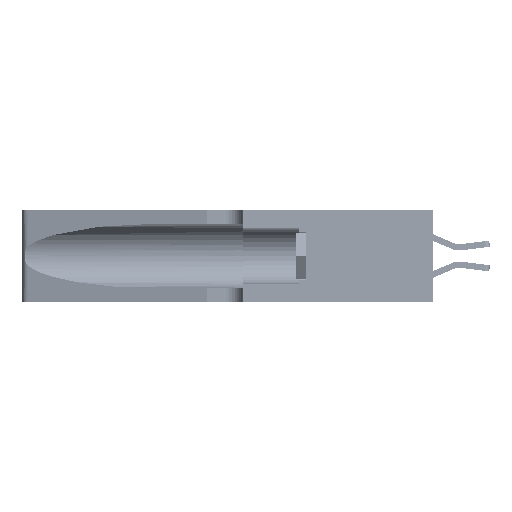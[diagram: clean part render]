
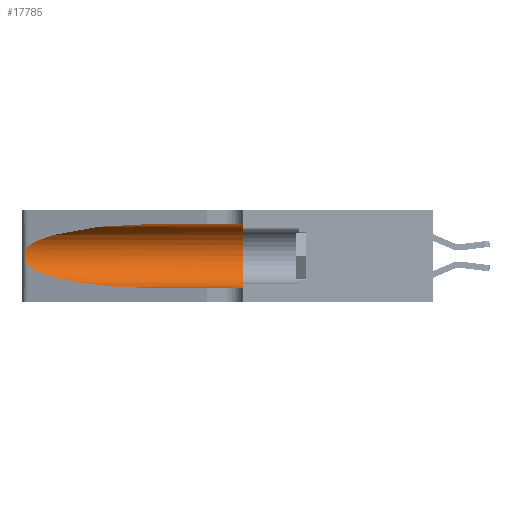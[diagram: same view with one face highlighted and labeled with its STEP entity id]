
A CAD part, left-side view. The second image highlights one B-rep face of the part: STEP entity #17785.
In plain terms, the highlighted cylindrical face has radius 3.308 mm (diameter 6.617 mm), a partial arc.
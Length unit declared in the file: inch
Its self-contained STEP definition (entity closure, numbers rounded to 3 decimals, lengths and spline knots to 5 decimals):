
#427 = CARTESIAN_POINT ( 'NONE',  ( 0.1305, 0.72297, 0.31525 ) ) ;
#527 = CARTESIAN_POINT ( 'NONE',  ( 0.25555, 1.22994, 0.2215 ) ) ;
#668 = CARTESIAN_POINT ( 'NONE',  ( 0.25639, 1.23186, 0.15144 ) ) ;
#2680 = ORIENTED_EDGE ( 'NONE', *, *, #5935, .T. ) ;
#2803 = LINE ( 'NONE', #15591, #28106 ) ;
#2886 = CARTESIAN_POINT ( 'NONE',  ( 0.1305, 0.72297, 0.31525 ) ) ;
#3024 = CARTESIAN_POINT ( 'NONE',  ( 0.1305, 1.61858, 0.185 ) ) ;
#3301 = CARTESIAN_POINT ( 'NONE',  ( 0.1305, 1.61858, 0.31525 ) ) ;
#3978 = CARTESIAN_POINT ( 'NONE',  ( 0.25487, 1.22718, 0.14631 ) ) ;
#4431 = ORIENTED_EDGE ( 'NONE', *, *, #32751, .T. ) ;
#5935 = EDGE_CURVE ( 'NONE', #42609, #28794, #17053, .T. ) ;
#6057 = EDGE_CURVE ( 'NONE', #17908, #11179, #16021, .T. ) ;
#7171 = CARTESIAN_POINT ( 'NONE',  ( 0.25639, 1.23184, 0.21858 ) ) ;
#8977 = ORIENTED_EDGE ( 'NONE', *, *, #35096, .F. ) ;
#9567 = CARTESIAN_POINT ( 'NONE',  ( 0.25487, 1.22718, 0.14631 ) ) ;
#10486 = CARTESIAN_POINT ( 'NONE',  ( 0.25854, 1.2359, 0.20912 ) ) ;
#10755 = DIRECTION ( 'NONE',  ( 0., 1., 0. ) ) ;
#10928 = ORIENTED_EDGE ( 'NONE', *, *, #6057, .T. ) ;
#11179 = VERTEX_POINT ( 'NONE', #24197 ) ;
#12167 = CARTESIAN_POINT ( 'NONE',  ( 0.18966, 0.96281, 0.05475 ) ) ;
#13814 = CARTESIAN_POINT ( 'NONE',  ( 0.26075, 1.23896, 0.19203 ) ) ;
#14240 = VECTOR ( 'NONE', #32155, 39.37008 ) ;
#15591 = CARTESIAN_POINT ( 'NONE',  ( 0.1305, 1.61858, 0.05475 ) ) ;
#16021 =( BOUNDED_CURVE ( )  B_SPLINE_CURVE ( 3, ( #2886, #42428, #22691, #26008 ),
 .UNSPECIFIED., .F., .T. ) 
 B_SPLINE_CURVE_WITH_KNOTS ( ( 4, 4 ),
 ( 1.5708, 2.84003 ),
 .UNSPECIFIED. ) 
 CURVE ( )  GEOMETRIC_REPRESENTATION_ITEM ( )  RATIONAL_B_SPLINE_CURVE ( ( 1., 0.87, 0.87, 1. ) ) 
 REPRESENTATION_ITEM ( '' )  );
#17053 =( BOUNDED_CURVE ( )  B_SPLINE_CURVE ( 3, ( #18861, #38571, #12167, #41848 ),
 .UNSPECIFIED., .F., .F. ) 
 B_SPLINE_CURVE_WITH_KNOTS ( ( 4, 4 ),
 ( 3.44316, 4.71239 ),
 .UNSPECIFIED. ) 
 CURVE ( )  GEOMETRIC_REPRESENTATION_ITEM ( )  RATIONAL_B_SPLINE_CURVE ( ( 1., 0.87, 0.87, 1. ) ) 
 REPRESENTATION_ITEM ( '' )  );
#17177 = CARTESIAN_POINT ( 'NONE',  ( 0.26017, 1.23833, 0.17102 ) ) ;
#17785 = ADVANCED_FACE ( 'NONE', ( #29604 ), #28546, .F. ) ;
#17908 = VERTEX_POINT ( 'NONE', #427 ) ;
#18273 = VERTEX_POINT ( 'NONE', #18518 ) ;
#18367 = AXIS2_PLACEMENT_3D ( 'NONE', #3024, #26150, #22841 ) ;
#18518 = CARTESIAN_POINT ( 'NONE',  ( 0.1305, 0.35, 0.05475 ) ) ;
#18861 = CARTESIAN_POINT ( 'NONE',  ( 0.25487, 1.22718, 0.14631 ) ) ;
#19488 = CARTESIAN_POINT ( 'NONE',  ( 0.1305, 0.72297, 0.05475 ) ) ;
#20491 = CARTESIAN_POINT ( 'NONE',  ( 0.25789, 1.23486, 0.15765 ) ) ;
#22110 = ORIENTED_EDGE ( 'NONE', *, *, #39446, .T. ) ;
#22691 = CARTESIAN_POINT ( 'NONE',  ( 0.2373, 1.15595, 0.28018 ) ) ;
#22841 = DIRECTION ( 'NONE',  ( 0., 0., -1. ) ) ;
#23023 = LINE ( 'NONE', #3301, #14240 ) ;
#23626 = CARTESIAN_POINT ( 'NONE',  ( 0.25487, 1.22718, 0.22369 ) ) ;
#23767 = CARTESIAN_POINT ( 'NONE',  ( 0.25555, 1.22993, 0.14849 ) ) ;
#24197 = CARTESIAN_POINT ( 'NONE',  ( 0.25487, 1.22718, 0.22369 ) ) ;
#24255 = AXIS2_PLACEMENT_3D ( 'NONE', #30521, #10755, #33857 ) ;
#25385 = DIRECTION ( 'NONE',  ( 0., -1., 0. ) ) ;
#25420 = CARTESIAN_POINT ( 'NONE',  ( 0.1305, 0.35, 0.31525 ) ) ;
#26008 = CARTESIAN_POINT ( 'NONE',  ( 0.25487, 1.22718, 0.22369 ) ) ;
#26150 = DIRECTION ( 'NONE',  ( 0., -1., 0. ) ) ;
#26974 = ORIENTED_EDGE ( 'NONE', *, *, #35434, .F. ) ;
#28106 = VECTOR ( 'NONE', #25385, 39.37008 ) ;
#28546 = CYLINDRICAL_SURFACE ( 'NONE', #18367, 0.13025 ) ;
#28794 = VERTEX_POINT ( 'NONE', #19488 ) ;
#29604 = FACE_OUTER_BOUND ( 'NONE', #42206, .T. ) ;
#29832 = VERTEX_POINT ( 'NONE', #25420 ) ;
#30276 = CARTESIAN_POINT ( 'NONE',  ( 0.25787, 1.23484, 0.2124 ) ) ;
#30521 = CARTESIAN_POINT ( 'NONE',  ( 0.1305, 0.35, 0.185 ) ) ;
#32155 = DIRECTION ( 'NONE',  ( 0., -1., 0. ) ) ;
#32751 = EDGE_CURVE ( 'NONE', #11179, #42609, #35545, .T. ) ;
#33599 = CARTESIAN_POINT ( 'NONE',  ( 0.26018, 1.23835, 0.19895 ) ) ;
#33857 = DIRECTION ( 'NONE',  ( 0., 0., 1. ) ) ;
#35096 = EDGE_CURVE ( 'NONE', #17908, #29832, #23023, .T. ) ;
#35434 = EDGE_CURVE ( 'NONE', #29832, #18273, #36947, .T. ) ;
#35545 = B_SPLINE_CURVE_WITH_KNOTS ( 'NONE', 3,
 ( #23626, #527, #7171, #30276, #10486, #33599, #13814, #36926, #17177, #40218, #20491, #668, #23767, #3978 ),
 .UNSPECIFIED., .F., .F.,
 ( 4, 2, 2, 2, 2, 2, 4 ),
 ( 0., 0.00027, 0.00053, 0.00107, 0.0016, 0.00187, 0.00214 ),
 .UNSPECIFIED. ) ;
#36926 = CARTESIAN_POINT ( 'NONE',  ( 0.26075, 1.23896, 0.178 ) ) ;
#36947 = CIRCLE ( 'NONE', #24255, 0.13025 ) ;
#38571 = CARTESIAN_POINT ( 'NONE',  ( 0.2373, 1.15595, 0.08982 ) ) ;
#39446 = EDGE_CURVE ( 'NONE', #28794, #18273, #2803, .T. ) ;
#40218 = CARTESIAN_POINT ( 'NONE',  ( 0.25856, 1.23593, 0.16098 ) ) ;
#41848 = CARTESIAN_POINT ( 'NONE',  ( 0.1305, 0.72297, 0.05475 ) ) ;
#42206 = EDGE_LOOP ( 'NONE', ( #10928, #4431, #2680, #22110, #26974, #8977 ) ) ;
#42428 = CARTESIAN_POINT ( 'NONE',  ( 0.18966, 0.96281, 0.31525 ) ) ;
#42609 = VERTEX_POINT ( 'NONE', #9567 ) ;
